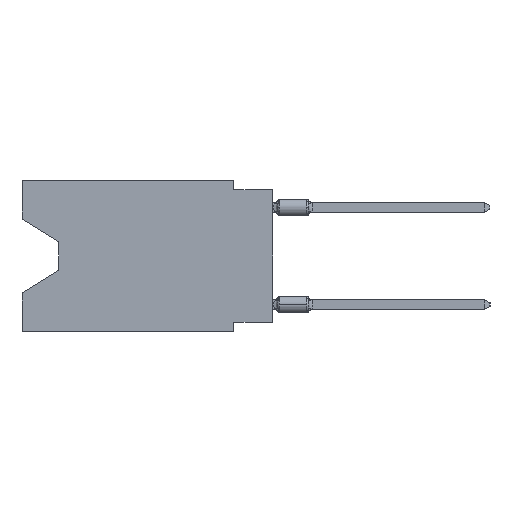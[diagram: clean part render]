
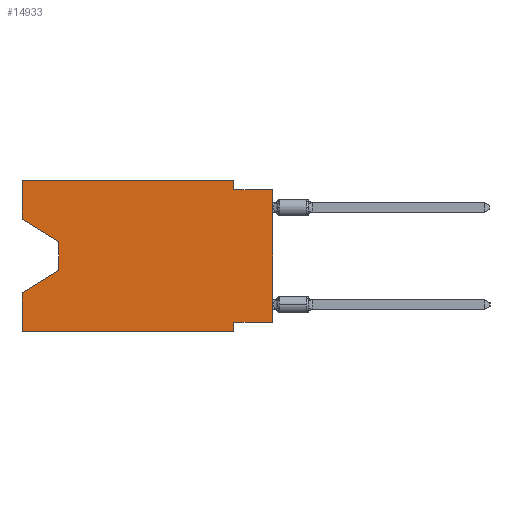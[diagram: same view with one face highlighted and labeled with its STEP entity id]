
A CAD part, left-side view. The second image highlights one B-rep face of the part: STEP entity #14933.
In plain terms, the highlighted planar face has unit normal (-1, 0, 0).
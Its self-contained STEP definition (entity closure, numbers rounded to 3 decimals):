
#781 = ORIENTED_EDGE ( 'NONE', *, *, #23851, .F. ) ;
#819 = VERTEX_POINT ( 'NONE', #28754 ) ;
#923 = ORIENTED_EDGE ( 'NONE', *, *, #17419, .F. ) ;
#1133 = DIRECTION ( 'NONE',  ( 0., 0., -1. ) ) ;
#1490 = CARTESIAN_POINT ( 'NONE',  ( 0., 13.97, -4.013 ) ) ;
#1651 = VERTEX_POINT ( 'NONE', #17427 ) ;
#1846 = LINE ( 'NONE', #19235, #15558 ) ;
#2250 = VECTOR ( 'NONE', #15668, 1000. ) ;
#2409 = CARTESIAN_POINT ( 'NONE',  ( 0., 13.97, -5.893 ) ) ;
#2467 = DIRECTION ( 'NONE',  ( 0., -1., 0. ) ) ;
#2496 = DIRECTION ( 'NONE',  ( 0., 0., -1. ) ) ;
#2682 = CARTESIAN_POINT ( 'NONE',  ( 0., 13.97, -5.893 ) ) ;
#2883 = ORIENTED_EDGE ( 'NONE', *, *, #5031, .T. ) ;
#3004 = VECTOR ( 'NONE', #22511, 1000. ) ;
#3691 = VECTOR ( 'NONE', #10035, 1000. ) ;
#4159 = LINE ( 'NONE', #24824, #3004 ) ;
#4960 = LINE ( 'NONE', #30868, #10678 ) ;
#5031 = EDGE_CURVE ( 'NONE', #15418, #33211, #19192, .T. ) ;
#5957 = LINE ( 'NONE', #18103, #37231 ) ;
#6088 = VERTEX_POINT ( 'NONE', #29920 ) ;
#7214 = CARTESIAN_POINT ( 'NONE',  ( 0., 2.54, -9.271 ) ) ;
#9835 = EDGE_CURVE ( 'NONE', #6088, #12714, #4159, .T. ) ;
#10035 = DIRECTION ( 'NONE',  ( 0., 0., -1. ) ) ;
#10060 = VERTEX_POINT ( 'NONE', #32907 ) ;
#10678 = VECTOR ( 'NONE', #31623, 1000. ) ;
#11007 = VERTEX_POINT ( 'NONE', #22130 ) ;
#11185 = DIRECTION ( 'NONE',  ( 1., 0., 0. ) ) ;
#12631 = DIRECTION ( 'NONE',  ( 0., -1., 0. ) ) ;
#12714 = VERTEX_POINT ( 'NONE', #25543 ) ;
#12918 = ORIENTED_EDGE ( 'NONE', *, *, #13608, .T. ) ;
#13023 = DIRECTION ( 'NONE',  ( 0., 1., 0. ) ) ;
#13195 = DIRECTION ( 'NONE',  ( 0., -0.855, -0.519 ) ) ;
#13608 = EDGE_CURVE ( 'NONE', #33211, #28338, #19122, .T. ) ;
#14101 = FACE_OUTER_BOUND ( 'NONE', #36246, .T. ) ;
#14220 = ORIENTED_EDGE ( 'NONE', *, *, #27405, .T. ) ;
#14933 = ADVANCED_FACE ( 'NONE', ( #14101 ), #17189, .F. ) ;
#15307 = LINE ( 'NONE', #24383, #2250 ) ;
#15418 = VERTEX_POINT ( 'NONE', #19348 ) ;
#15432 = CARTESIAN_POINT ( 'NONE',  ( 0., 2.54, 0. ) ) ;
#15558 = VECTOR ( 'NONE', #28140, 1000. ) ;
#15668 = DIRECTION ( 'NONE',  ( 0., 0., -1. ) ) ;
#15825 = LINE ( 'NONE', #15432, #34667 ) ;
#16494 = ORIENTED_EDGE ( 'NONE', *, *, #24377, .F. ) ;
#16888 = VERTEX_POINT ( 'NONE', #20448 ) ;
#16954 = LINE ( 'NONE', #17336, #32807 ) ;
#17189 = PLANE ( 'NONE',  #21049 ) ;
#17336 = CARTESIAN_POINT ( 'NONE',  ( 0., 16.383, 0. ) ) ;
#17419 = EDGE_CURVE ( 'NONE', #15418, #1651, #5957, .T. ) ;
#17427 = CARTESIAN_POINT ( 'NONE',  ( 0., 16.383, 0. ) ) ;
#17953 = EDGE_CURVE ( 'NONE', #819, #23471, #33723, .T. ) ;
#18103 = CARTESIAN_POINT ( 'NONE',  ( 0., 16.383, 0. ) ) ;
#19122 = LINE ( 'NONE', #22041, #3691 ) ;
#19192 = LINE ( 'NONE', #21538, #26920 ) ;
#19235 = CARTESIAN_POINT ( 'NONE',  ( 0., 16.383, 0. ) ) ;
#19263 = ORIENTED_EDGE ( 'NONE', *, *, #24075, .F. ) ;
#19348 = CARTESIAN_POINT ( 'NONE',  ( 0., 16.383, -2.546 ) ) ;
#20448 = CARTESIAN_POINT ( 'NONE',  ( 0., 2.54, 0. ) ) ;
#20738 = EDGE_CURVE ( 'NONE', #11007, #24772, #24996, .T. ) ;
#21049 = AXIS2_PLACEMENT_3D ( 'NONE', #37672, #11185, #2496 ) ;
#21120 = DIRECTION ( 'NONE',  ( 0., 0.855, -0.519 ) ) ;
#21204 = DIRECTION ( 'NONE',  ( 0., 0., 1. ) ) ;
#21538 = CARTESIAN_POINT ( 'NONE',  ( 0., 16.383, -2.546 ) ) ;
#22041 = CARTESIAN_POINT ( 'NONE',  ( 0., 13.97, -4.013 ) ) ;
#22130 = CARTESIAN_POINT ( 'NONE',  ( 0., 2.54, -0.635 ) ) ;
#22511 = DIRECTION ( 'NONE',  ( 0., -1., 0. ) ) ;
#22527 = VECTOR ( 'NONE', #12631, 1000. ) ;
#23471 = VERTEX_POINT ( 'NONE', #7214 ) ;
#23851 = EDGE_CURVE ( 'NONE', #16888, #11007, #15825, .T. ) ;
#23952 = ORIENTED_EDGE ( 'NONE', *, *, #9835, .T. ) ;
#24075 = EDGE_CURVE ( 'NONE', #1651, #16888, #16954, .T. ) ;
#24377 = EDGE_CURVE ( 'NONE', #6088, #10060, #1846, .T. ) ;
#24383 = CARTESIAN_POINT ( 'NONE',  ( 0., 2.54, -9.906 ) ) ;
#24772 = VERTEX_POINT ( 'NONE', #28461 ) ;
#24824 = CARTESIAN_POINT ( 'NONE',  ( 0., 16.383, -9.906 ) ) ;
#24996 = LINE ( 'NONE', #36788, #22527 ) ;
#25337 = ORIENTED_EDGE ( 'NONE', *, *, #34235, .F. ) ;
#25543 = CARTESIAN_POINT ( 'NONE',  ( 0., 2.54, -9.906 ) ) ;
#26920 = VECTOR ( 'NONE', #13195, 1000. ) ;
#27405 = EDGE_CURVE ( 'NONE', #28338, #10060, #28889, .T. ) ;
#28140 = DIRECTION ( 'NONE',  ( 0., 0., 1. ) ) ;
#28338 = VERTEX_POINT ( 'NONE', #2682 ) ;
#28461 = CARTESIAN_POINT ( 'NONE',  ( 0., 0., -0.635 ) ) ;
#28487 = EDGE_CURVE ( 'NONE', #819, #24772, #4960, .T. ) ;
#28715 = ORIENTED_EDGE ( 'NONE', *, *, #28487, .T. ) ;
#28754 = CARTESIAN_POINT ( 'NONE',  ( 0., 0., -9.271 ) ) ;
#28889 = LINE ( 'NONE', #2409, #34106 ) ;
#29920 = CARTESIAN_POINT ( 'NONE',  ( 0., 16.383, -9.906 ) ) ;
#30868 = CARTESIAN_POINT ( 'NONE',  ( 0., 0., 0. ) ) ;
#31623 = DIRECTION ( 'NONE',  ( 0., 0., 1. ) ) ;
#32807 = VECTOR ( 'NONE', #2467, 1000. ) ;
#32907 = CARTESIAN_POINT ( 'NONE',  ( 0., 16.383, -7.36 ) ) ;
#33015 = ORIENTED_EDGE ( 'NONE', *, *, #20738, .F. ) ;
#33211 = VERTEX_POINT ( 'NONE', #1490 ) ;
#33723 = LINE ( 'NONE', #36600, #34781 ) ;
#34106 = VECTOR ( 'NONE', #21120, 1000. ) ;
#34235 = EDGE_CURVE ( 'NONE', #23471, #12714, #15307, .T. ) ;
#34667 = VECTOR ( 'NONE', #1133, 1000. ) ;
#34781 = VECTOR ( 'NONE', #13023, 1000. ) ;
#35256 = ORIENTED_EDGE ( 'NONE', *, *, #17953, .F. ) ;
#36246 = EDGE_LOOP ( 'NONE', ( #2883, #12918, #14220, #16494, #23952, #25337, #35256, #28715, #33015, #781, #19263, #923 ) ) ;
#36600 = CARTESIAN_POINT ( 'NONE',  ( 0., 0., -9.271 ) ) ;
#36788 = CARTESIAN_POINT ( 'NONE',  ( 0., 0., -0.635 ) ) ;
#37231 = VECTOR ( 'NONE', #21204, 1000. ) ;
#37672 = CARTESIAN_POINT ( 'NONE',  ( 0., 16.383, 0. ) ) ;
